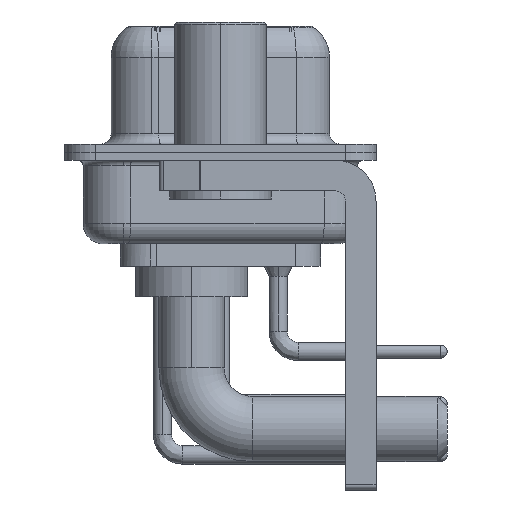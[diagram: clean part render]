
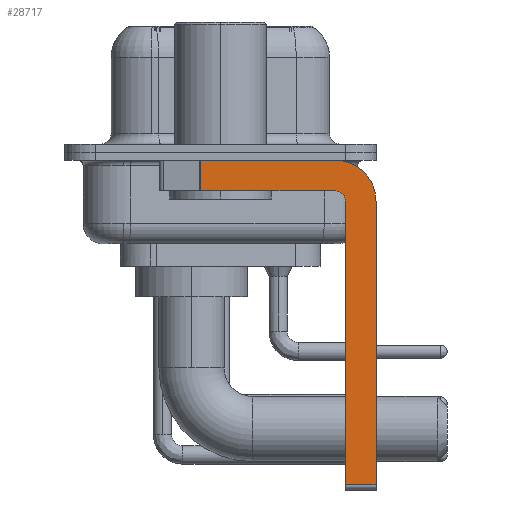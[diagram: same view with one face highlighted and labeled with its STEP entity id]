
A CAD part, left-side view. The second image highlights one B-rep face of the part: STEP entity #28717.
In plain terms, the highlighted planar face has unit normal (-1, 0, 0).
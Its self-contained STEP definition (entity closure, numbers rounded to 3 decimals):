
#12 = CIRCLE ( 'NONE', #14910, 0.5 ) ;
#1079 = PLANE ( 'NONE',  #29949 ) ;
#1770 = ORIENTED_EDGE ( 'NONE', *, *, #20476, .T. ) ;
#1780 = VERTEX_POINT ( 'NONE', #22647 ) ;
#2170 = CIRCLE ( 'NONE', #15027, 2. ) ;
#3108 = DIRECTION ( 'NONE',  ( 0., -1., 0. ) ) ;
#3164 = CARTESIAN_POINT ( 'NONE',  ( -2.9, -5.65, -2.4 ) ) ;
#3431 = CARTESIAN_POINT ( 'NONE',  ( -2.9, -5.65, -0.4 ) ) ;
#3692 = CARTESIAN_POINT ( 'NONE',  ( -2.9, -5.65, -2.4 ) ) ;
#4209 = EDGE_CURVE ( 'NONE', #29754, #13088, #21350, .T. ) ;
#4611 = CARTESIAN_POINT ( 'NONE',  ( -2.9, -6.15, -16.35 ) ) ;
#4625 = CARTESIAN_POINT ( 'NONE',  ( -2.9, 0.978, -1.9 ) ) ;
#5113 = DIRECTION ( 'NONE',  ( 1., 0., 0. ) ) ;
#5834 = ORIENTED_EDGE ( 'NONE', *, *, #11004, .T. ) ;
#5909 = ORIENTED_EDGE ( 'NONE', *, *, #6696, .F. ) ;
#6264 = VERTEX_POINT ( 'NONE', #3431 ) ;
#6606 = ORIENTED_EDGE ( 'NONE', *, *, #30285, .F. ) ;
#6696 = EDGE_CURVE ( 'NONE', #19559, #13279, #27544, .T. ) ;
#6777 = ORIENTED_EDGE ( 'NONE', *, *, #11821, .F. ) ;
#6988 = CARTESIAN_POINT ( 'NONE',  ( -2.9, 3., -0.4 ) ) ;
#7033 = DIRECTION ( 'NONE',  ( 0., 0., 1. ) ) ;
#9456 = CARTESIAN_POINT ( 'NONE',  ( -2.9, -5.65, -2.4 ) ) ;
#9710 = VECTOR ( 'NONE', #26639, 1000. ) ;
#10630 = DIRECTION ( 'NONE',  ( 0., 1., 0. ) ) ;
#11004 = EDGE_CURVE ( 'NONE', #29842, #13279, #11495, .T. ) ;
#11495 = LINE ( 'NONE', #19066, #9710 ) ;
#11821 = EDGE_CURVE ( 'NONE', #13088, #19559, #12, .T. ) ;
#12295 = DIRECTION ( 'NONE',  ( 0., -1., 0. ) ) ;
#12774 = DIRECTION ( 'NONE',  ( 0., 0., -1. ) ) ;
#13088 = VERTEX_POINT ( 'NONE', #15897 ) ;
#13279 = VERTEX_POINT ( 'NONE', #4625 ) ;
#13515 = DIRECTION ( 'NONE',  ( -1., 0., 0. ) ) ;
#14910 = AXIS2_PLACEMENT_3D ( 'NONE', #3692, #13515, #18507 ) ;
#15022 = LINE ( 'NONE', #27747, #18717 ) ;
#15027 = AXIS2_PLACEMENT_3D ( 'NONE', #9456, #5113, #26846 ) ;
#15737 = VECTOR ( 'NONE', #10630, 1000. ) ;
#15897 = CARTESIAN_POINT ( 'NONE',  ( -2.9, -6.15, -2.4 ) ) ;
#15939 = CARTESIAN_POINT ( 'NONE',  ( -2.9, -5.65, -1.9 ) ) ;
#16347 = VECTOR ( 'NONE', #3108, 1000. ) ;
#17456 = EDGE_CURVE ( 'NONE', #1780, #24558, #15022, .T. ) ;
#17762 = LINE ( 'NONE', #27581, #16347 ) ;
#18507 = DIRECTION ( 'NONE',  ( 0., 0., 1. ) ) ;
#18717 = VECTOR ( 'NONE', #12774, 1000. ) ;
#18783 = CARTESIAN_POINT ( 'NONE',  ( -2.9, -6.15, -16.6 ) ) ;
#19066 = CARTESIAN_POINT ( 'NONE',  ( -2.9, 0.978, -1.9 ) ) ;
#19322 = EDGE_LOOP ( 'NONE', ( #6606, #5834, #5909, #6777, #26722, #1770, #23742, #25461 ) ) ;
#19559 = VERTEX_POINT ( 'NONE', #23820 ) ;
#20476 = EDGE_CURVE ( 'NONE', #29754, #24558, #17762, .T. ) ;
#20695 = DIRECTION ( 'NONE',  ( 1., 0., 0. ) ) ;
#21340 = CARTESIAN_POINT ( 'NONE',  ( -2.9, -7.65, -16.35 ) ) ;
#21350 = LINE ( 'NONE', #18783, #22545 ) ;
#21782 = LINE ( 'NONE', #6988, #26951 ) ;
#22545 = VECTOR ( 'NONE', #7033, 1000. ) ;
#22647 = CARTESIAN_POINT ( 'NONE',  ( -2.9, -7.65, -2.4 ) ) ;
#23138 = FACE_OUTER_BOUND ( 'NONE', #19322, .T. ) ;
#23742 = ORIENTED_EDGE ( 'NONE', *, *, #17456, .F. ) ;
#23820 = CARTESIAN_POINT ( 'NONE',  ( -2.9, -5.65, -1.9 ) ) ;
#24558 = VERTEX_POINT ( 'NONE', #21340 ) ;
#25461 = ORIENTED_EDGE ( 'NONE', *, *, #27163, .F. ) ;
#26639 = DIRECTION ( 'NONE',  ( 0., 0., -1. ) ) ;
#26722 = ORIENTED_EDGE ( 'NONE', *, *, #4209, .F. ) ;
#26846 = DIRECTION ( 'NONE',  ( 0., 0., -1. ) ) ;
#26951 = VECTOR ( 'NONE', #12295, 1000. ) ;
#27163 = EDGE_CURVE ( 'NONE', #6264, #1780, #2170, .T. ) ;
#27544 = LINE ( 'NONE', #15939, #15737 ) ;
#27581 = CARTESIAN_POINT ( 'NONE',  ( -2.9, -5.65, -16.35 ) ) ;
#27747 = CARTESIAN_POINT ( 'NONE',  ( -2.9, -7.65, -2.4 ) ) ;
#28279 = DIRECTION ( 'NONE',  ( 0., 0., -1. ) ) ;
#28717 = ADVANCED_FACE ( 'NONE', ( #23138 ), #1079, .F. ) ;
#29566 = CARTESIAN_POINT ( 'NONE',  ( -2.9, 0.978, -0.4 ) ) ;
#29754 = VERTEX_POINT ( 'NONE', #4611 ) ;
#29842 = VERTEX_POINT ( 'NONE', #29566 ) ;
#29949 = AXIS2_PLACEMENT_3D ( 'NONE', #3164, #20695, #28279 ) ;
#30285 = EDGE_CURVE ( 'NONE', #29842, #6264, #21782, .T. ) ;
